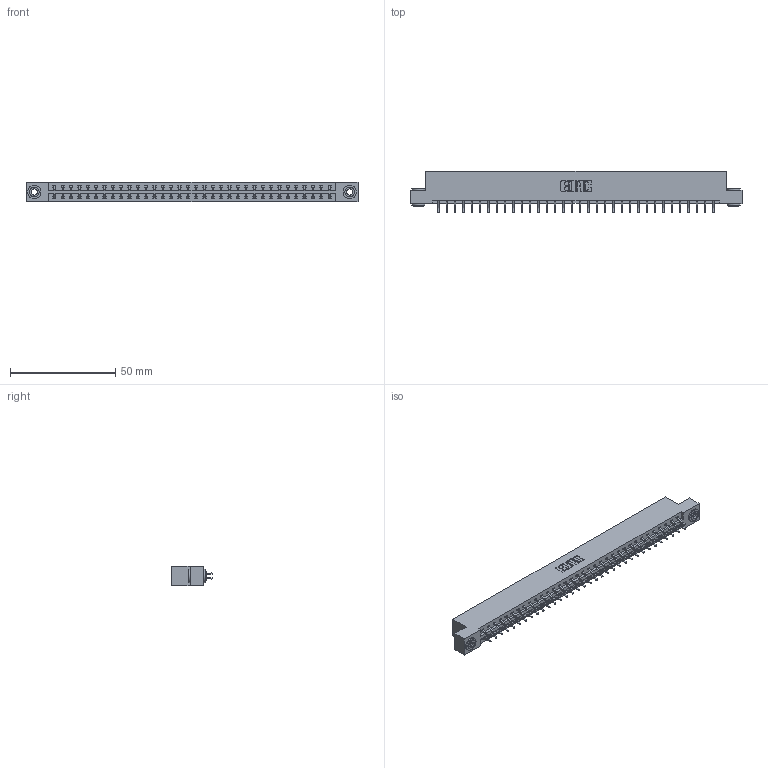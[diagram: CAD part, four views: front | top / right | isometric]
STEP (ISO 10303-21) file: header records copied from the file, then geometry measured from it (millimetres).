
FILE_DESCRIPTION (( 'STEP AP203' ), '1' );
FILE_NAME ('387-068-556-203.STEP', '2019-10-19T21:44:58', ( '' ), ( '' ), 'SwSTEP 2.0', 'SolidWorks 2016', '' );
FILE_SCHEMA (( 'CONFIG_CONTROL_DESIGN' ));
Length unit declared in the file: inch
Products named in the file (4): 387-068-556-203; 337 Part_Flush Mounting Lugs - 0.156 Dia-TH; 345-292-001_556 Tail; 345-250-002_345-250-002-102
Assembly tree (71 placements, depth 2):
  387-068-556-203
    337 Part_Flush Mounting Lugs - 0.156 Dia-TH
    345-292-001_556 Tail  x68
    345-250-002_345-250-002-102  x2
Bounding box: 157.73 x 19.57 x 9.4 mm (x, y, z)
Volume: 16533.5 mm3; surface area: 18766.1 mm2
Topology: 71 solids, 71 shells, 4232 faces, 12559 edges, 8278 vertices
Faces by surface type: plane 2936, cylinder 1288, cone 8
Entity records: 28266 total; most frequent: CARTESIAN_POINT 4757, ORIENTED_EDGE 4674, DIRECTION 4083, EDGE_CURVE 2337, LINE 2177, VECTOR 2177, VERTEX_POINT 1554, AXIS2_PLACEMENT_3D 953
